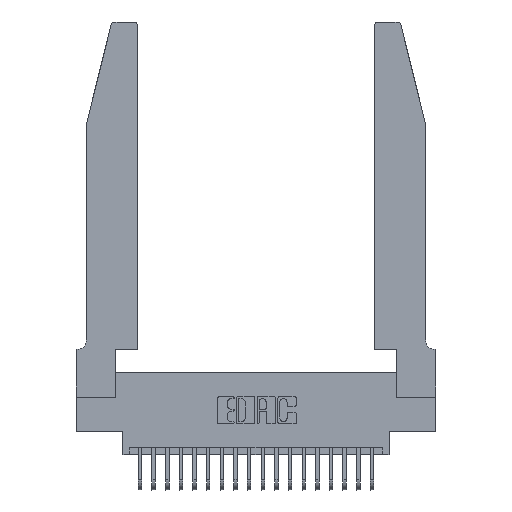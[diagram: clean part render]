
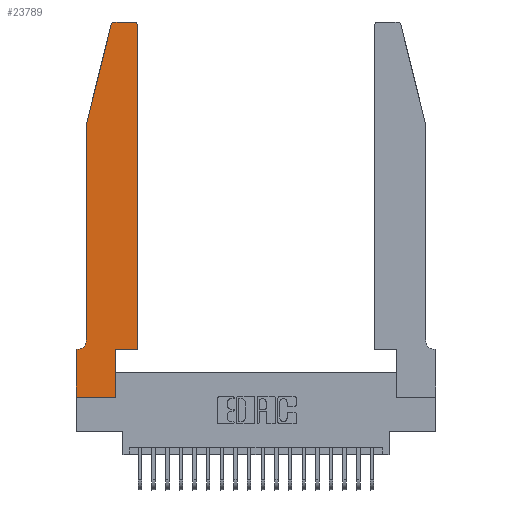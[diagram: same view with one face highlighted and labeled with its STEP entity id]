
A CAD part, top view. The second image highlights one B-rep face of the part: STEP entity #23789.
In plain terms, the highlighted planar face has unit normal (0, 0, 1).
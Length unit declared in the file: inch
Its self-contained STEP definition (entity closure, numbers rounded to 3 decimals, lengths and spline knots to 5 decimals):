
#302 = EDGE_CURVE ( 'NONE', #4519, #20216, #16055, .T. ) ;
#799 = AXIS2_PLACEMENT_3D ( 'NONE', #18579, #20427, #9370 ) ;
#921 = DIRECTION ( 'NONE',  ( 0., 0., 1. ) ) ;
#1021 = VECTOR ( 'NONE', #1450, 39.37008 ) ;
#1450 = DIRECTION ( 'NONE',  ( 0., 1., 0. ) ) ;
#2005 = DIRECTION ( 'NONE',  ( 1., 0., 0. ) ) ;
#2067 = CARTESIAN_POINT ( 'NONE',  ( 0.0755, 2., 0.37 ) ) ;
#2094 = LINE ( 'NONE', #7497, #22878 ) ;
#2131 = DIRECTION ( 'NONE',  ( 0., 1., 0. ) ) ;
#2256 = EDGE_CURVE ( 'NONE', #16824, #7304, #2094, .T. ) ;
#2344 = EDGE_LOOP ( 'NONE', ( #23884, #8632, #4460, #3456, #13672, #22049, #20268, #13801, #23206, #19178, #9332, #21038 ) ) ;
#2544 = EDGE_CURVE ( 'NONE', #20216, #5303, #4613, .T. ) ;
#2545 = CARTESIAN_POINT ( 'NONE',  ( 0., 0.35, 0.37 ) ) ;
#3456 = ORIENTED_EDGE ( 'NONE', *, *, #20619, .T. ) ;
#3789 = EDGE_CURVE ( 'NONE', #12311, #4519, #20494, .T. ) ;
#3994 = EDGE_CURVE ( 'NONE', #19103, #12311, #17322, .T. ) ;
#4460 = ORIENTED_EDGE ( 'NONE', *, *, #18314, .T. ) ;
#4511 = VERTEX_POINT ( 'NONE', #12922 ) ;
#4519 = VERTEX_POINT ( 'NONE', #17155 ) ;
#4613 = LINE ( 'NONE', #20662, #13927 ) ;
#4644 = CARTESIAN_POINT ( 'NONE',  ( 0.0755, 2., 0.37 ) ) ;
#5194 = VECTOR ( 'NONE', #10587, 39.37008 ) ;
#5303 = VERTEX_POINT ( 'NONE', #15379 ) ;
#5368 = CARTESIAN_POINT ( 'NONE',  ( 0.4205, 2.72, 0.37 ) ) ;
#5409 = LINE ( 'NONE', #4644, #5991 ) ;
#5434 = CARTESIAN_POINT ( 'NONE',  ( 0., 0.35, 0.37 ) ) ;
#5589 = EDGE_CURVE ( 'NONE', #14526, #16824, #23436, .T. ) ;
#5653 = LINE ( 'NONE', #22540, #13211 ) ;
#5991 = VECTOR ( 'NONE', #6609, 39.37008 ) ;
#6482 = VECTOR ( 'NONE', #17139, 39.37008 ) ;
#6609 = DIRECTION ( 'NONE',  ( -0.239, -0.971, 0. ) ) ;
#7304 = VERTEX_POINT ( 'NONE', #11762 ) ;
#7497 = CARTESIAN_POINT ( 'NONE',  ( 0.2605, 2.75, 0.37 ) ) ;
#7768 = CARTESIAN_POINT ( 'NONE',  ( 0.0755, 2., 0.37 ) ) ;
#7826 = CARTESIAN_POINT ( 'NONE',  ( 0.4205, 2.75, 0.37 ) ) ;
#7950 = EDGE_CURVE ( 'NONE', #9525, #14905, #14148, .T. ) ;
#8034 = CARTESIAN_POINT ( 'NONE',  ( 0.2865, 0.35, 0.37 ) ) ;
#8632 = ORIENTED_EDGE ( 'NONE', *, *, #16508, .T. ) ;
#9332 = ORIENTED_EDGE ( 'NONE', *, *, #9546, .T. ) ;
#9370 = DIRECTION ( 'NONE',  ( -1., 0., 0. ) ) ;
#9525 = VERTEX_POINT ( 'NONE', #13378 ) ;
#9546 = EDGE_CURVE ( 'NONE', #5303, #14526, #5653, .T. ) ;
#9897 = DIRECTION ( 'NONE',  ( 1., 0., 0. ) ) ;
#10185 = DIRECTION ( 'NONE',  ( 1., 0., 0. ) ) ;
#10587 = DIRECTION ( 'NONE',  ( -1., 0., 0. ) ) ;
#10675 = CARTESIAN_POINT ( 'NONE',  ( 0.0755, 0.35, 0.37 ) ) ;
#10724 = CARTESIAN_POINT ( 'NONE',  ( 0., 0., 0.37 ) ) ;
#10920 = DIRECTION ( 'NONE',  ( 1., 0., 0. ) ) ;
#10997 = CARTESIAN_POINT ( 'NONE',  ( 0., 0., 0.37 ) ) ;
#11038 = LINE ( 'NONE', #10675, #5194 ) ;
#11241 = DIRECTION ( 'NONE',  ( 1., 0., 0. ) ) ;
#11460 = DIRECTION ( 'NONE',  ( 0., 0., 1. ) ) ;
#11762 = CARTESIAN_POINT ( 'NONE',  ( 0.284, 2.75, 0.37 ) ) ;
#11976 = CARTESIAN_POINT ( 'NONE',  ( 0.284, 2.72, 0.37 ) ) ;
#12008 = PLANE ( 'NONE',  #15475 ) ;
#12311 = VERTEX_POINT ( 'NONE', #10724 ) ;
#12565 = CARTESIAN_POINT ( 'NONE',  ( 0.2865, 0.35, 0.37 ) ) ;
#12922 = CARTESIAN_POINT ( 'NONE',  ( 0.25487, 2.72718, 0.37 ) ) ;
#13211 = VECTOR ( 'NONE', #2131, 39.37008 ) ;
#13378 = CARTESIAN_POINT ( 'NONE',  ( 0.0755, 0.42, 0.37 ) ) ;
#13672 = ORIENTED_EDGE ( 'NONE', *, *, #7950, .T. ) ;
#13801 = ORIENTED_EDGE ( 'NONE', *, *, #3789, .T. ) ;
#13927 = VECTOR ( 'NONE', #11241, 39.37008 ) ;
#14051 = DIRECTION ( 'NONE',  ( -1., 0., 0. ) ) ;
#14148 = CIRCLE ( 'NONE', #799, 0.07 ) ;
#14344 = LINE ( 'NONE', #7768, #6482 ) ;
#14526 = VERTEX_POINT ( 'NONE', #22250 ) ;
#14905 = VERTEX_POINT ( 'NONE', #16206 ) ;
#15379 = CARTESIAN_POINT ( 'NONE',  ( 0.4505, 0.35, 0.37 ) ) ;
#15475 = AXIS2_PLACEMENT_3D ( 'NONE', #2545, #921, #9897 ) ;
#15614 = VECTOR ( 'NONE', #10920, 39.37008 ) ;
#16009 = DIRECTION ( 'NONE',  ( 0., 0., 1. ) ) ;
#16055 = LINE ( 'NONE', #12565, #1021 ) ;
#16089 = AXIS2_PLACEMENT_3D ( 'NONE', #11976, #16009, #10185 ) ;
#16206 = CARTESIAN_POINT ( 'NONE',  ( 0.0055, 0.35, 0.37 ) ) ;
#16508 = EDGE_CURVE ( 'NONE', #7304, #4511, #21589, .T. ) ;
#16824 = VERTEX_POINT ( 'NONE', #7826 ) ;
#16889 = CARTESIAN_POINT ( 'NONE',  ( 0., 0., 0.37 ) ) ;
#17139 = DIRECTION ( 'NONE',  ( 0., -1., 0. ) ) ;
#17155 = CARTESIAN_POINT ( 'NONE',  ( 0.2865, 0., 0.37 ) ) ;
#17322 = LINE ( 'NONE', #16889, #19914 ) ;
#17932 = FACE_OUTER_BOUND ( 'NONE', #2344, .T. ) ;
#18314 = EDGE_CURVE ( 'NONE', #4511, #23586, #5409, .T. ) ;
#18579 = CARTESIAN_POINT ( 'NONE',  ( 0.0055, 0.42, 0.37 ) ) ;
#18979 = DIRECTION ( 'NONE',  ( 0., -1., 0. ) ) ;
#19103 = VERTEX_POINT ( 'NONE', #5434 ) ;
#19178 = ORIENTED_EDGE ( 'NONE', *, *, #2544, .T. ) ;
#19347 = AXIS2_PLACEMENT_3D ( 'NONE', #5368, #11460, #2005 ) ;
#19914 = VECTOR ( 'NONE', #18979, 39.37008 ) ;
#20216 = VERTEX_POINT ( 'NONE', #8034 ) ;
#20268 = ORIENTED_EDGE ( 'NONE', *, *, #3994, .T. ) ;
#20427 = DIRECTION ( 'NONE',  ( 0., 0., -1. ) ) ;
#20494 = LINE ( 'NONE', #10997, #15614 ) ;
#20619 = EDGE_CURVE ( 'NONE', #23586, #9525, #14344, .T. ) ;
#20662 = CARTESIAN_POINT ( 'NONE',  ( 0.4505, 0.35, 0.37 ) ) ;
#21038 = ORIENTED_EDGE ( 'NONE', *, *, #5589, .T. ) ;
#21589 = CIRCLE ( 'NONE', #16089, 0.03 ) ;
#22049 = ORIENTED_EDGE ( 'NONE', *, *, #22823, .T. ) ;
#22250 = CARTESIAN_POINT ( 'NONE',  ( 0.4505, 2.72, 0.37 ) ) ;
#22540 = CARTESIAN_POINT ( 'NONE',  ( 0.4505, 0.35, 0.37 ) ) ;
#22823 = EDGE_CURVE ( 'NONE', #14905, #19103, #11038, .T. ) ;
#22878 = VECTOR ( 'NONE', #14051, 39.37008 ) ;
#23206 = ORIENTED_EDGE ( 'NONE', *, *, #302, .T. ) ;
#23436 = CIRCLE ( 'NONE', #19347, 0.03 ) ;
#23586 = VERTEX_POINT ( 'NONE', #2067 ) ;
#23789 = ADVANCED_FACE ( 'NONE', ( #17932 ), #12008, .T. ) ;
#23884 = ORIENTED_EDGE ( 'NONE', *, *, #2256, .T. ) ;
